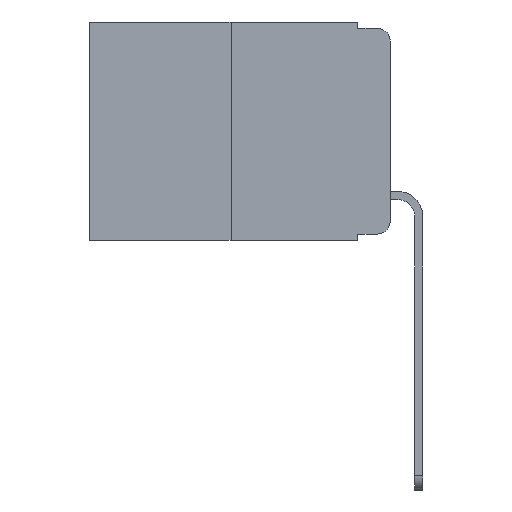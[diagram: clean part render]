
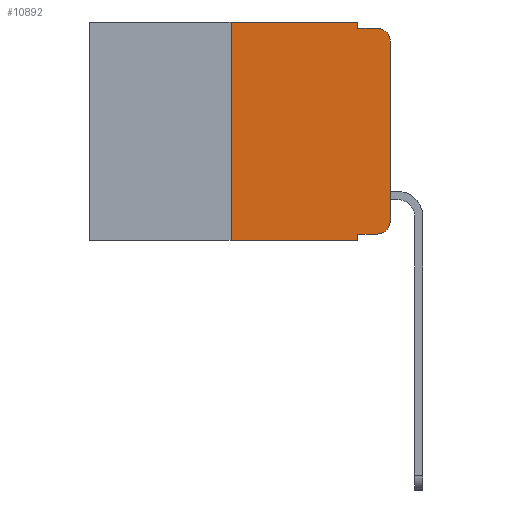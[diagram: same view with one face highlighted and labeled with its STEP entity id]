
A CAD part, left-side view. The second image highlights one B-rep face of the part: STEP entity #10892.
In plain terms, the highlighted planar face has unit normal (-1, 0, 0).
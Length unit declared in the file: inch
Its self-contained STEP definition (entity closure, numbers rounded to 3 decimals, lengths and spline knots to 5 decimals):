
#545 = VECTOR ( 'NONE', #7353, 39.37008 ) ;
#863 = CARTESIAN_POINT ( 'NONE',  ( 0., 0., 0. ) ) ;
#982 = DIRECTION ( 'NONE',  ( 0., 0., -1. ) ) ;
#1144 = VECTOR ( 'NONE', #3596, 39.37008 ) ;
#1534 = VECTOR ( 'NONE', #10635, 39.37008 ) ;
#1589 = VERTEX_POINT ( 'NONE', #12151 ) ;
#1930 = CIRCLE ( 'NONE', #4061, 0.02 ) ;
#2077 = EDGE_LOOP ( 'NONE', ( #11891, #4149, #6883, #9501, #7524, #5177, #13030, #13602, #11740, #6738 ) ) ;
#2142 = DIRECTION ( 'NONE',  ( 0., 0., 1. ) ) ;
#2342 = CARTESIAN_POINT ( 'NONE',  ( 0., 0.051, 0. ) ) ;
#2449 = CARTESIAN_POINT ( 'NONE',  ( 0., 0.25, 0. ) ) ;
#2526 = AXIS2_PLACEMENT_3D ( 'NONE', #9592, #12596, #6661 ) ;
#2895 = VECTOR ( 'NONE', #11846, 39.37008 ) ;
#3596 = DIRECTION ( 'NONE',  ( 0., -1., 0. ) ) ;
#3705 = DIRECTION ( 'NONE',  ( 0., 0., 1. ) ) ;
#3849 = LINE ( 'NONE', #5365, #545 ) ;
#3909 = AXIS2_PLACEMENT_3D ( 'NONE', #12207, #6249, #13117 ) ;
#3966 = CARTESIAN_POINT ( 'NONE',  ( 0., 0., -0.03 ) ) ;
#4061 = AXIS2_PLACEMENT_3D ( 'NONE', #13449, #7604, #982 ) ;
#4149 = ORIENTED_EDGE ( 'NONE', *, *, #7007, .T. ) ;
#4347 = LINE ( 'NONE', #2342, #1534 ) ;
#4354 = VECTOR ( 'NONE', #11847, 39.37008 ) ;
#4652 = EDGE_CURVE ( 'NONE', #12791, #12539, #12056, .T. ) ;
#5030 = VECTOR ( 'NONE', #2142, 39.37008 ) ;
#5100 = VERTEX_POINT ( 'NONE', #13357 ) ;
#5177 = ORIENTED_EDGE ( 'NONE', *, *, #7298, .F. ) ;
#5365 = CARTESIAN_POINT ( 'NONE',  ( 0., 0.473, 0. ) ) ;
#5556 = FACE_OUTER_BOUND ( 'NONE', #2077, .T. ) ;
#5569 = VERTEX_POINT ( 'NONE', #3966 ) ;
#5995 = CIRCLE ( 'NONE', #3909, 0.02 ) ;
#6249 = DIRECTION ( 'NONE',  ( -1., 0., 0. ) ) ;
#6371 = VERTEX_POINT ( 'NONE', #12668 ) ;
#6469 = CARTESIAN_POINT ( 'NONE',  ( 0., 0.051, -0.01 ) ) ;
#6521 = VERTEX_POINT ( 'NONE', #6964 ) ;
#6661 = DIRECTION ( 'NONE',  ( 0., 0., -1. ) ) ;
#6738 = ORIENTED_EDGE ( 'NONE', *, *, #7871, .T. ) ;
#6837 = EDGE_CURVE ( 'NONE', #5100, #1589, #3849, .T. ) ;
#6883 = ORIENTED_EDGE ( 'NONE', *, *, #7188, .F. ) ;
#6964 = CARTESIAN_POINT ( 'NONE',  ( 0., 0.02, -0.01 ) ) ;
#6984 = EDGE_CURVE ( 'NONE', #6371, #5569, #7694, .T. ) ;
#7007 = EDGE_CURVE ( 'NONE', #5569, #6521, #1930, .T. ) ;
#7012 = VERTEX_POINT ( 'NONE', #9544 ) ;
#7149 = CARTESIAN_POINT ( 'NONE',  ( 0., 0.051, -0.333 ) ) ;
#7188 = EDGE_CURVE ( 'NONE', #10236, #6521, #9689, .T. ) ;
#7213 = EDGE_CURVE ( 'NONE', #1589, #10236, #4347, .T. ) ;
#7215 = LINE ( 'NONE', #9977, #12486 ) ;
#7298 = EDGE_CURVE ( 'NONE', #12791, #5100, #12051, .T. ) ;
#7353 = DIRECTION ( 'NONE',  ( 0., -1., 0. ) ) ;
#7367 = EDGE_CURVE ( 'NONE', #9002, #12539, #11075, .T. ) ;
#7524 = ORIENTED_EDGE ( 'NONE', *, *, #6837, .F. ) ;
#7604 = DIRECTION ( 'NONE',  ( -1., 0., 0. ) ) ;
#7694 = LINE ( 'NONE', #863, #5030 ) ;
#7717 = EDGE_CURVE ( 'NONE', #9002, #7012, #7215, .T. ) ;
#7871 = EDGE_CURVE ( 'NONE', #7012, #6371, #5995, .T. ) ;
#8639 = PLANE ( 'NONE',  #2526 ) ;
#8707 = CARTESIAN_POINT ( 'NONE',  ( 0., 0.051, -0.01 ) ) ;
#8784 = VECTOR ( 'NONE', #3705, 39.37008 ) ;
#9002 = VERTEX_POINT ( 'NONE', #7149 ) ;
#9501 = ORIENTED_EDGE ( 'NONE', *, *, #7213, .F. ) ;
#9544 = CARTESIAN_POINT ( 'NONE',  ( 0., 0.02, -0.333 ) ) ;
#9592 = CARTESIAN_POINT ( 'NONE',  ( 0., 0.473, 0. ) ) ;
#9689 = LINE ( 'NONE', #8707, #1144 ) ;
#9728 = CARTESIAN_POINT ( 'NONE',  ( 0., 0.051, -0.343 ) ) ;
#9977 = CARTESIAN_POINT ( 'NONE',  ( 0., 0.051, -0.333 ) ) ;
#10031 = CARTESIAN_POINT ( 'NONE',  ( 0., 0.25, -0.343 ) ) ;
#10236 = VERTEX_POINT ( 'NONE', #6469 ) ;
#10635 = DIRECTION ( 'NONE',  ( 0., 0., -1. ) ) ;
#10771 = CARTESIAN_POINT ( 'NONE',  ( 0., 0.051, 0. ) ) ;
#10774 = CARTESIAN_POINT ( 'NONE',  ( 0., 0.473, -0.343 ) ) ;
#10892 = ADVANCED_FACE ( 'NONE', ( #5556 ), #8639, .F. ) ;
#11075 = LINE ( 'NONE', #10771, #2895 ) ;
#11740 = ORIENTED_EDGE ( 'NONE', *, *, #7717, .T. ) ;
#11846 = DIRECTION ( 'NONE',  ( 0., 0., -1. ) ) ;
#11847 = DIRECTION ( 'NONE',  ( 0., -1., 0. ) ) ;
#11891 = ORIENTED_EDGE ( 'NONE', *, *, #6984, .T. ) ;
#12008 = DIRECTION ( 'NONE',  ( 0., -1., 0. ) ) ;
#12051 = LINE ( 'NONE', #2449, #8784 ) ;
#12056 = LINE ( 'NONE', #10774, #4354 ) ;
#12151 = CARTESIAN_POINT ( 'NONE',  ( 0., 0.051, 0. ) ) ;
#12207 = CARTESIAN_POINT ( 'NONE',  ( 0., 0.02, -0.313 ) ) ;
#12486 = VECTOR ( 'NONE', #12008, 39.37008 ) ;
#12539 = VERTEX_POINT ( 'NONE', #9728 ) ;
#12596 = DIRECTION ( 'NONE',  ( 1., 0., 0. ) ) ;
#12668 = CARTESIAN_POINT ( 'NONE',  ( 0., 0., -0.313 ) ) ;
#12791 = VERTEX_POINT ( 'NONE', #10031 ) ;
#13030 = ORIENTED_EDGE ( 'NONE', *, *, #4652, .T. ) ;
#13117 = DIRECTION ( 'NONE',  ( 0., 0., -1. ) ) ;
#13357 = CARTESIAN_POINT ( 'NONE',  ( 0., 0.25, 0. ) ) ;
#13449 = CARTESIAN_POINT ( 'NONE',  ( 0., 0.02, -0.03 ) ) ;
#13602 = ORIENTED_EDGE ( 'NONE', *, *, #7367, .F. ) ;
